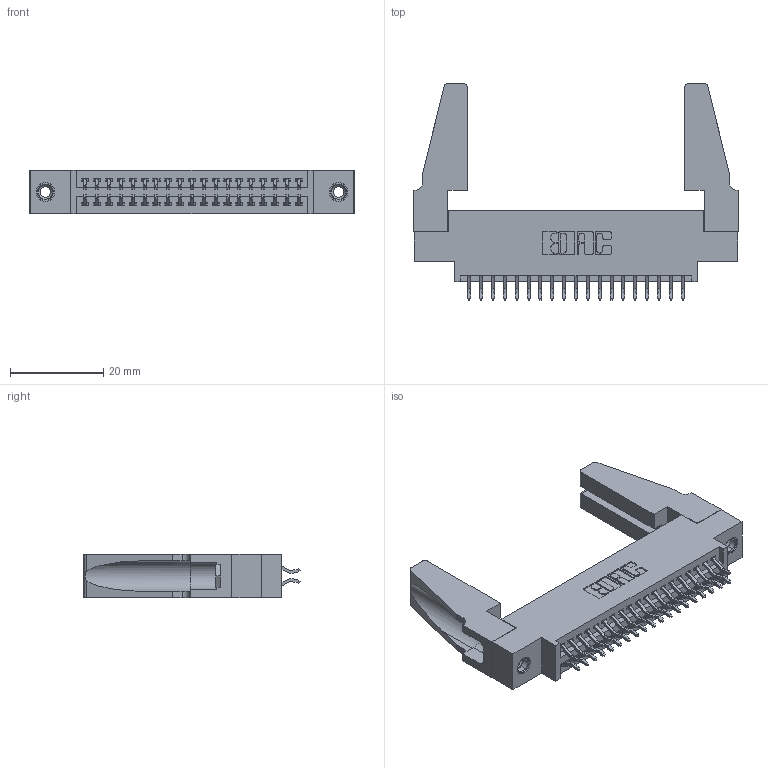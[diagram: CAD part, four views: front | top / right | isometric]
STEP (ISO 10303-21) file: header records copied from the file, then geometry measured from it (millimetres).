
FILE_DESCRIPTION (( 'STEP AP203' ), '1' );
FILE_NAME ('395-038-556-888.STEP', '2019-10-18T04:25:36', ( '' ), ( '' ), 'SwSTEP 2.0', 'SolidWorks 2016', '' );
FILE_SCHEMA (( 'CONFIG_CONTROL_DESIGN' ));
Length unit declared in the file: inch
Products named in the file (5): 345 Part_0.170 Offset - 0.156 Dia-TH; 345-292-001_556 Tail; 345-250-001_345-250-001-102; 345-220-078_345-220-088; 395-038-556-888
Assembly tree (43 placements, depth 2):
  395-038-556-888
    345 Part_0.170 Offset - 0.156 Dia-TH
    345-292-001_556 Tail  x38
    345-250-001_345-250-001-102  x2
    345-220-078_345-220-088  x2
Bounding box: 69.49 x 46.41 x 9.4 mm (x, y, z)
Volume: 9674.8 mm3; surface area: 12280.2 mm2
Topology: 43 solids, 43 shells, 2382 faces, 7013 edges, 4614 vertices
Faces by surface type: plane 1562, cylinder 804, cone 12, torus 4
Entity records: 20504 total; most frequent: CARTESIAN_POINT 3470, ORIENTED_EDGE 3352, DIRECTION 3080, EDGE_CURVE 1676, LINE 1418, VECTOR 1418, VERTEX_POINT 1110, AXIS2_PLACEMENT_3D 831
